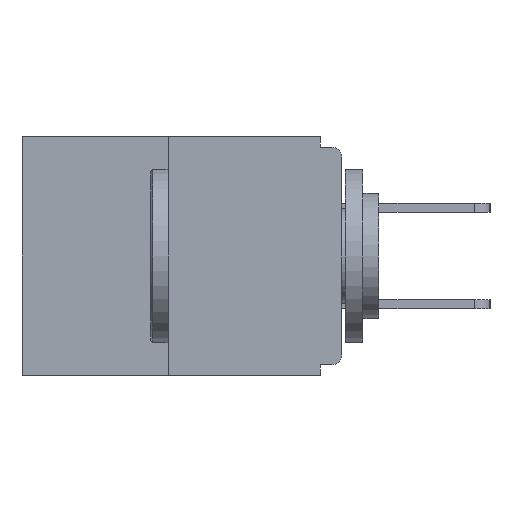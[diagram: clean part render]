
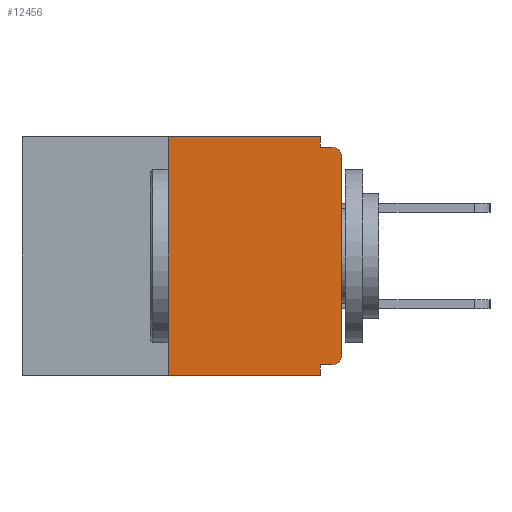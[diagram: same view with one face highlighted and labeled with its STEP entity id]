
A CAD part, left-side view. The second image highlights one B-rep face of the part: STEP entity #12456.
In plain terms, the highlighted planar face has unit normal (-1, 0, 0).
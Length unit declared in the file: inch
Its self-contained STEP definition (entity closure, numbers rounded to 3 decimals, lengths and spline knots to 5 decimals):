
#515 = VERTEX_POINT ( 'NONE', #8997 ) ;
#1229 = DIRECTION ( 'NONE',  ( 0., -1., 0. ) ) ;
#1556 = VERTEX_POINT ( 'NONE', #5793 ) ;
#2101 = DIRECTION ( 'NONE',  ( 0., 0., -1. ) ) ;
#2206 = VECTOR ( 'NONE', #2662, 39.37008 ) ;
#2376 = DIRECTION ( 'NONE',  ( 0., 0., -1. ) ) ;
#2482 = EDGE_LOOP ( 'NONE', ( #4810, #7743, #6111, #8961, #17051, #17688, #2992, #5336, #8558, #10408 ) ) ;
#2587 = VERTEX_POINT ( 'NONE', #11576 ) ;
#2622 = CARTESIAN_POINT ( 'NONE',  ( 0., 0.46, 0. ) ) ;
#2662 = DIRECTION ( 'NONE',  ( 0., 0., 1. ) ) ;
#2668 = LINE ( 'NONE', #14888, #4538 ) ;
#2992 = ORIENTED_EDGE ( 'NONE', *, *, #5527, .T. ) ;
#3164 = CARTESIAN_POINT ( 'NONE',  ( 0., 0.46, 0. ) ) ;
#3361 = DIRECTION ( 'NONE',  ( 1., 0., 0. ) ) ;
#3585 = VECTOR ( 'NONE', #18529, 39.37008 ) ;
#3609 = CARTESIAN_POINT ( 'NONE',  ( 0., 0.031, -0.328 ) ) ;
#3943 = DIRECTION ( 'NONE',  ( 0., -1., 0. ) ) ;
#3995 = CIRCLE ( 'NONE', #5183, 0.015 ) ;
#4150 = EDGE_CURVE ( 'NONE', #515, #11507, #19448, .T. ) ;
#4222 = LINE ( 'NONE', #8866, #5669 ) ;
#4538 = VECTOR ( 'NONE', #11927, 39.37008 ) ;
#4773 = VECTOR ( 'NONE', #16215, 39.37008 ) ;
#4810 = ORIENTED_EDGE ( 'NONE', *, *, #4150, .F. ) ;
#5183 = AXIS2_PLACEMENT_3D ( 'NONE', #11269, #15782, #2101 ) ;
#5336 = ORIENTED_EDGE ( 'NONE', *, *, #7796, .T. ) ;
#5337 = VECTOR ( 'NONE', #3943, 39.37008 ) ;
#5527 = EDGE_CURVE ( 'NONE', #2587, #13465, #18925, .T. ) ;
#5548 = EDGE_CURVE ( 'NONE', #14816, #11141, #6705, .T. ) ;
#5669 = VECTOR ( 'NONE', #13350, 39.37008 ) ;
#5793 = CARTESIAN_POINT ( 'NONE',  ( 0., 0.031, -0.343 ) ) ;
#6087 = PLANE ( 'NONE',  #11767 ) ;
#6111 = ORIENTED_EDGE ( 'NONE', *, *, #15710, .T. ) ;
#6340 = DIRECTION ( 'NONE',  ( 0., 0., -1. ) ) ;
#6470 = CARTESIAN_POINT ( 'NONE',  ( 0., 0.031, -0.015 ) ) ;
#6705 = LINE ( 'NONE', #19332, #4773 ) ;
#6891 = DIRECTION ( 'NONE',  ( -1., 0., 0. ) ) ;
#6921 = LINE ( 'NONE', #8010, #3585 ) ;
#7743 = ORIENTED_EDGE ( 'NONE', *, *, #12774, .F. ) ;
#7796 = EDGE_CURVE ( 'NONE', #13465, #11141, #3995, .T. ) ;
#8010 = CARTESIAN_POINT ( 'NONE',  ( 0., 0., -0.328 ) ) ;
#8358 = EDGE_CURVE ( 'NONE', #11507, #14816, #4222, .T. ) ;
#8492 = LINE ( 'NONE', #18294, #17432 ) ;
#8548 = CARTESIAN_POINT ( 'NONE',  ( 0., 0., 0. ) ) ;
#8558 = ORIENTED_EDGE ( 'NONE', *, *, #5548, .F. ) ;
#8722 = EDGE_CURVE ( 'NONE', #10438, #1556, #8492, .T. ) ;
#8866 = CARTESIAN_POINT ( 'NONE',  ( 0., 0.031, 0. ) ) ;
#8961 = ORIENTED_EDGE ( 'NONE', *, *, #8722, .F. ) ;
#8997 = CARTESIAN_POINT ( 'NONE',  ( 0., 0.25, 0. ) ) ;
#9638 = LINE ( 'NONE', #19034, #10090 ) ;
#9833 = AXIS2_PLACEMENT_3D ( 'NONE', #12814, #6891, #2376 ) ;
#10090 = VECTOR ( 'NONE', #1229, 39.37008 ) ;
#10408 = ORIENTED_EDGE ( 'NONE', *, *, #8358, .F. ) ;
#10438 = VERTEX_POINT ( 'NONE', #3609 ) ;
#10970 = CARTESIAN_POINT ( 'NONE',  ( 0., 0.015, -0.015 ) ) ;
#11141 = VERTEX_POINT ( 'NONE', #10970 ) ;
#11269 = CARTESIAN_POINT ( 'NONE',  ( 0., 0.015, -0.03 ) ) ;
#11507 = VERTEX_POINT ( 'NONE', #11919 ) ;
#11576 = CARTESIAN_POINT ( 'NONE',  ( 0., 0., -0.313 ) ) ;
#11767 = AXIS2_PLACEMENT_3D ( 'NONE', #3164, #3361, #16985 ) ;
#11843 = VERTEX_POINT ( 'NONE', #15915 ) ;
#11919 = CARTESIAN_POINT ( 'NONE',  ( 0., 0.031, 0. ) ) ;
#11927 = DIRECTION ( 'NONE',  ( 0., 0., 1. ) ) ;
#12456 = ADVANCED_FACE ( 'NONE', ( #13466 ), #6087, .F. ) ;
#12694 = CARTESIAN_POINT ( 'NONE',  ( 0., 0., -0.03 ) ) ;
#12774 = EDGE_CURVE ( 'NONE', #11843, #515, #2668, .T. ) ;
#12814 = CARTESIAN_POINT ( 'NONE',  ( 0., 0.015, -0.313 ) ) ;
#13350 = DIRECTION ( 'NONE',  ( 0., 0., -1. ) ) ;
#13394 = EDGE_CURVE ( 'NONE', #17715, #10438, #6921, .T. ) ;
#13465 = VERTEX_POINT ( 'NONE', #12694 ) ;
#13466 = FACE_OUTER_BOUND ( 'NONE', #2482, .T. ) ;
#14399 = CARTESIAN_POINT ( 'NONE',  ( 0., 0.015, -0.328 ) ) ;
#14816 = VERTEX_POINT ( 'NONE', #6470 ) ;
#14888 = CARTESIAN_POINT ( 'NONE',  ( 0., 0.25, 0. ) ) ;
#15452 = CIRCLE ( 'NONE', #9833, 0.015 ) ;
#15710 = EDGE_CURVE ( 'NONE', #11843, #1556, #9638, .T. ) ;
#15782 = DIRECTION ( 'NONE',  ( -1., 0., 0. ) ) ;
#15915 = CARTESIAN_POINT ( 'NONE',  ( 0., 0.25, -0.343 ) ) ;
#16215 = DIRECTION ( 'NONE',  ( 0., -1., 0. ) ) ;
#16985 = DIRECTION ( 'NONE',  ( 0., 0., -1. ) ) ;
#17051 = ORIENTED_EDGE ( 'NONE', *, *, #13394, .F. ) ;
#17170 = EDGE_CURVE ( 'NONE', #17715, #2587, #15452, .T. ) ;
#17432 = VECTOR ( 'NONE', #6340, 39.37008 ) ;
#17688 = ORIENTED_EDGE ( 'NONE', *, *, #17170, .T. ) ;
#17715 = VERTEX_POINT ( 'NONE', #14399 ) ;
#18294 = CARTESIAN_POINT ( 'NONE',  ( 0., 0.031, -0.343 ) ) ;
#18529 = DIRECTION ( 'NONE',  ( 0., 1., 0. ) ) ;
#18925 = LINE ( 'NONE', #8548, #2206 ) ;
#19034 = CARTESIAN_POINT ( 'NONE',  ( 0., 0.46, -0.343 ) ) ;
#19332 = CARTESIAN_POINT ( 'NONE',  ( 0., 0., -0.015 ) ) ;
#19448 = LINE ( 'NONE', #2622, #5337 ) ;
